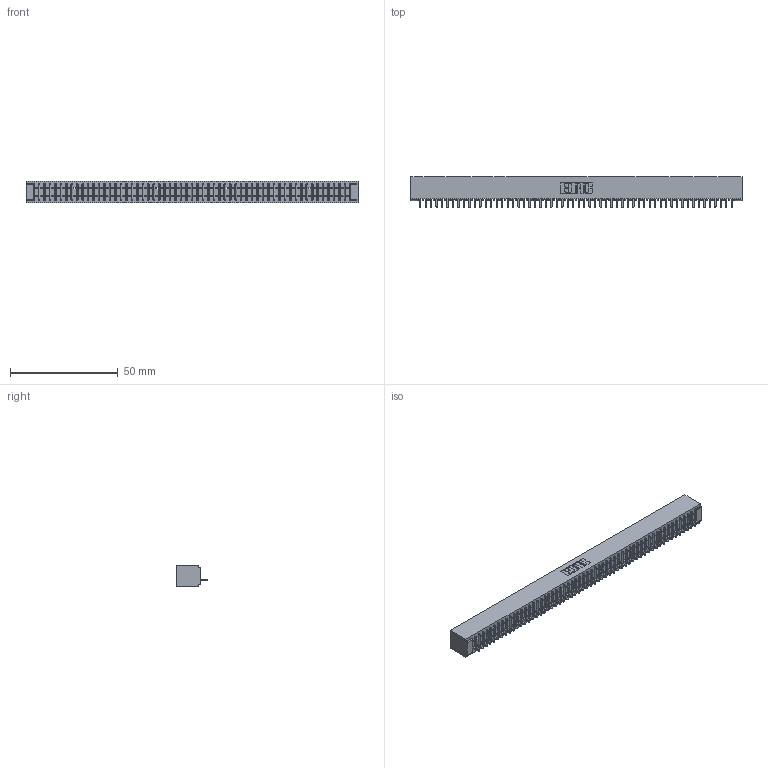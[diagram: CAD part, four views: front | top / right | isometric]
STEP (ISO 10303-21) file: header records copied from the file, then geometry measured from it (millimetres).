
FILE_DESCRIPTION (( 'STEP AP203' ), '1' );
FILE_NAME ('391-058-520-101.STEP', '2018-08-09T11:35:29', ( '' ), ( '' ), 'SwSTEP 2.0', 'SolidWorks 2016', '' );
FILE_SCHEMA (( 'CONFIG_CONTROL_DESIGN' ));
Length unit declared in the file: inch
Products named in the file (3): 341-292-001_341-292-120; 391-058-520-101; 341 Part_No Mounting Lugs
Assembly tree (59 placements, depth 2):
  391-058-520-101
    341 Part_No Mounting Lugs
    341-292-001_341-292-120  x58
Bounding box: 154.31 x 14.27 x 10.16 mm (x, y, z)
Volume: 11231.8 mm3; surface area: 18162.7 mm2
Topology: 59 solids, 59 shells, 4864 faces, 14038 edges, 9006 vertices
Faces by surface type: plane 3022, cylinder 1610, sphere 118, torus 114
Entity records: 65927 total; most frequent: CARTESIAN_POINT 11208, ORIENTED_EDGE 11196, DIRECTION 10804, EDGE_CURVE 5598, VECTOR 4544, LINE 4544, VERTEX_POINT 3534, AXIS2_PLACEMENT_3D 3130
